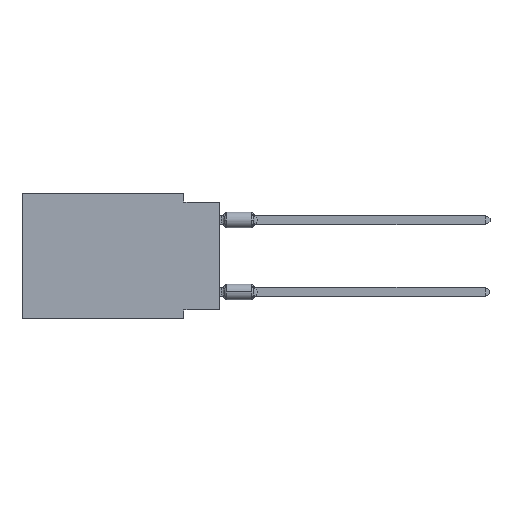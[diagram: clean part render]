
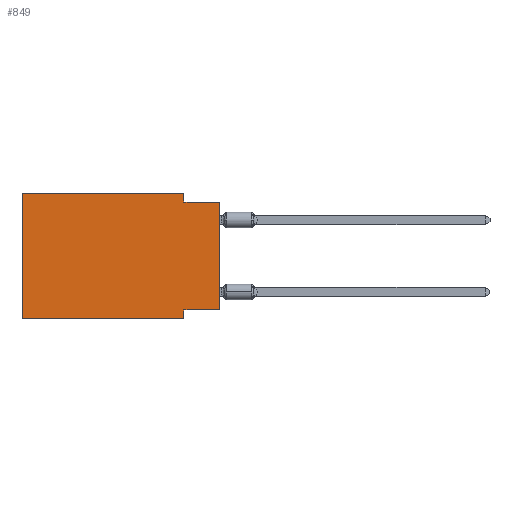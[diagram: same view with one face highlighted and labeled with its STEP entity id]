
A CAD part, left-side view. The second image highlights one B-rep face of the part: STEP entity #849.
In plain terms, the highlighted planar face has unit normal (-1, 0, 0).
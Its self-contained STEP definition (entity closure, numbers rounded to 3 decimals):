
#96 = VERTEX_POINT ( 'NONE', #8497 ) ;
#358 = LINE ( 'NONE', #1826, #5171 ) ;
#441 = CARTESIAN_POINT ( 'NONE',  ( 0., 2.54, 0. ) ) ;
#538 = CARTESIAN_POINT ( 'NONE',  ( 0., 13.97, 0. ) ) ;
#616 = CARTESIAN_POINT ( 'NONE',  ( 0., 13.97, 0. ) ) ;
#849 = ADVANCED_FACE ( 'NONE', ( #11078 ), #9715, .F. ) ;
#1684 = CARTESIAN_POINT ( 'NONE',  ( 0., 0., -8.255 ) ) ;
#1826 = CARTESIAN_POINT ( 'NONE',  ( 0., 0., 0. ) ) ;
#2015 = LINE ( 'NONE', #7526, #13379 ) ;
#2089 = DIRECTION ( 'NONE',  ( 0., 0., -1. ) ) ;
#2201 = LINE ( 'NONE', #9458, #8502 ) ;
#2728 = DIRECTION ( 'NONE',  ( 1., 0., 0. ) ) ;
#2735 = AXIS2_PLACEMENT_3D ( 'NONE', #15252, #2728, #18105 ) ;
#2998 = CARTESIAN_POINT ( 'NONE',  ( 0., 13.97, -8.89 ) ) ;
#3204 = DIRECTION ( 'NONE',  ( 0., 0., 1. ) ) ;
#3225 = VERTEX_POINT ( 'NONE', #9660 ) ;
#3400 = EDGE_CURVE ( 'NONE', #5394, #3723, #358, .T. ) ;
#3723 = VERTEX_POINT ( 'NONE', #7054 ) ;
#4453 = EDGE_LOOP ( 'NONE', ( #6846, #7024, #15843, #6524, #17831, #9785, #11330, #4854 ) ) ;
#4519 = VECTOR ( 'NONE', #6684, 1000. ) ;
#4575 = LINE ( 'NONE', #10180, #7472 ) ;
#4651 = EDGE_CURVE ( 'NONE', #3225, #3723, #2015, .T. ) ;
#4854 = ORIENTED_EDGE ( 'NONE', *, *, #7767, .F. ) ;
#5171 = VECTOR ( 'NONE', #3204, 1000. ) ;
#5394 = VERTEX_POINT ( 'NONE', #1684 ) ;
#5748 = VECTOR ( 'NONE', #9081, 1000. ) ;
#6218 = DIRECTION ( 'NONE',  ( 0., -1., 0. ) ) ;
#6318 = EDGE_CURVE ( 'NONE', #96, #3225, #7686, .T. ) ;
#6445 = EDGE_CURVE ( 'NONE', #12916, #96, #13175, .T. ) ;
#6522 = EDGE_CURVE ( 'NONE', #8454, #13981, #7874, .T. ) ;
#6524 = ORIENTED_EDGE ( 'NONE', *, *, #6445, .F. ) ;
#6684 = DIRECTION ( 'NONE',  ( 0., 0., -1. ) ) ;
#6846 = ORIENTED_EDGE ( 'NONE', *, *, #3400, .T. ) ;
#7024 = ORIENTED_EDGE ( 'NONE', *, *, #4651, .F. ) ;
#7054 = CARTESIAN_POINT ( 'NONE',  ( 0., 0., -0.635 ) ) ;
#7213 = CARTESIAN_POINT ( 'NONE',  ( 0., 2.54, -8.89 ) ) ;
#7472 = VECTOR ( 'NONE', #8894, 1000. ) ;
#7526 = CARTESIAN_POINT ( 'NONE',  ( 0., 0., -0.635 ) ) ;
#7686 = LINE ( 'NONE', #441, #17674 ) ;
#7767 = EDGE_CURVE ( 'NONE', #5394, #8454, #4575, .T. ) ;
#7874 = LINE ( 'NONE', #8058, #4519 ) ;
#8058 = CARTESIAN_POINT ( 'NONE',  ( 0., 2.54, -8.89 ) ) ;
#8454 = VERTEX_POINT ( 'NONE', #14889 ) ;
#8497 = CARTESIAN_POINT ( 'NONE',  ( 0., 2.54, 0. ) ) ;
#8502 = VECTOR ( 'NONE', #9275, 1000. ) ;
#8894 = DIRECTION ( 'NONE',  ( 0., 1., 0. ) ) ;
#9081 = DIRECTION ( 'NONE',  ( 0., 0., 1. ) ) ;
#9275 = DIRECTION ( 'NONE',  ( 0., -1., 0. ) ) ;
#9458 = CARTESIAN_POINT ( 'NONE',  ( 0., 13.97, -8.89 ) ) ;
#9660 = CARTESIAN_POINT ( 'NONE',  ( 0., 2.54, -0.635 ) ) ;
#9715 = PLANE ( 'NONE',  #2735 ) ;
#9785 = ORIENTED_EDGE ( 'NONE', *, *, #12180, .T. ) ;
#10180 = CARTESIAN_POINT ( 'NONE',  ( 0., 0., -8.255 ) ) ;
#10540 = DIRECTION ( 'NONE',  ( 0., -1., 0. ) ) ;
#11078 = FACE_OUTER_BOUND ( 'NONE', #4453, .T. ) ;
#11330 = ORIENTED_EDGE ( 'NONE', *, *, #6522, .F. ) ;
#12153 = VECTOR ( 'NONE', #6218, 1000. ) ;
#12180 = EDGE_CURVE ( 'NONE', #14013, #13981, #2201, .T. ) ;
#12916 = VERTEX_POINT ( 'NONE', #16027 ) ;
#13175 = LINE ( 'NONE', #616, #12153 ) ;
#13379 = VECTOR ( 'NONE', #10540, 1000. ) ;
#13981 = VERTEX_POINT ( 'NONE', #7213 ) ;
#14013 = VERTEX_POINT ( 'NONE', #2998 ) ;
#14889 = CARTESIAN_POINT ( 'NONE',  ( 0., 2.54, -8.255 ) ) ;
#15063 = EDGE_CURVE ( 'NONE', #14013, #12916, #15989, .T. ) ;
#15252 = CARTESIAN_POINT ( 'NONE',  ( 0., 13.97, 0. ) ) ;
#15843 = ORIENTED_EDGE ( 'NONE', *, *, #6318, .F. ) ;
#15989 = LINE ( 'NONE', #538, #5748 ) ;
#16027 = CARTESIAN_POINT ( 'NONE',  ( 0., 13.97, 0. ) ) ;
#17674 = VECTOR ( 'NONE', #2089, 1000. ) ;
#17831 = ORIENTED_EDGE ( 'NONE', *, *, #15063, .F. ) ;
#18105 = DIRECTION ( 'NONE',  ( 0., 0., -1. ) ) ;
